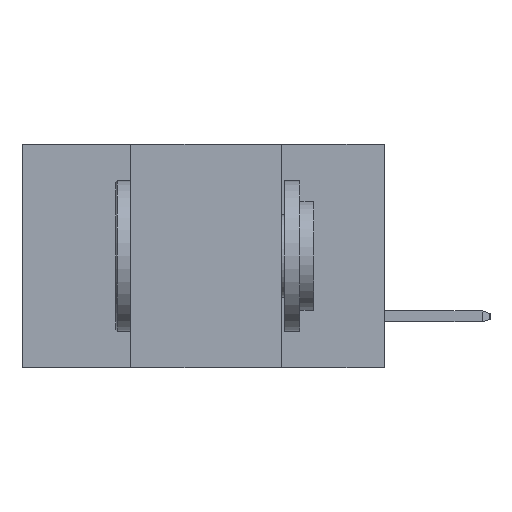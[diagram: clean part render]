
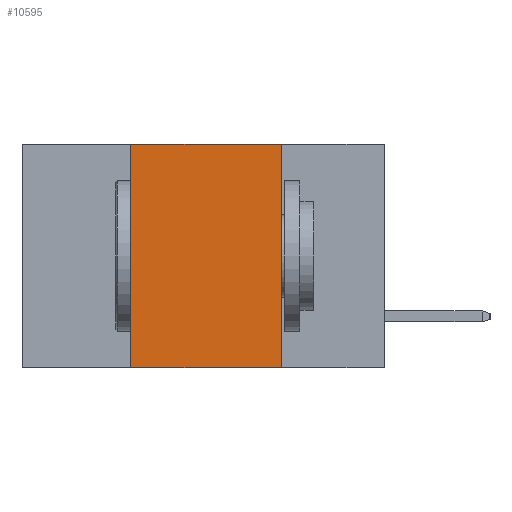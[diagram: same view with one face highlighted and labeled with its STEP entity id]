
A CAD part, left-side view. The second image highlights one B-rep face of the part: STEP entity #10595.
In plain terms, the highlighted planar face has unit normal (-1, 0, 0).
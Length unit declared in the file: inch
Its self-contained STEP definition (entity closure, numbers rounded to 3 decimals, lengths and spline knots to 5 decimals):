
#344 = ORIENTED_EDGE ( 'NONE', *, *, #7234, .F. ) ;
#406 = VERTEX_POINT ( 'NONE', #2446 ) ;
#418 = EDGE_CURVE ( 'NONE', #406, #7225, #11298, .T. ) ;
#929 = ORIENTED_EDGE ( 'NONE', *, *, #8746, .F. ) ;
#1268 = ORIENTED_EDGE ( 'NONE', *, *, #7599, .T. ) ;
#2446 = CARTESIAN_POINT ( 'NONE',  ( 0., 0.17, 0. ) ) ;
#2513 = LINE ( 'NONE', #8634, #9541 ) ;
#3117 = LINE ( 'NONE', #3710, #10073 ) ;
#3343 = DIRECTION ( 'NONE',  ( 0., -1., 0. ) ) ;
#3696 = CARTESIAN_POINT ( 'NONE',  ( 0., 0.17, 0. ) ) ;
#3710 = CARTESIAN_POINT ( 'NONE',  ( 0., 0.6, -0.37 ) ) ;
#3955 = AXIS2_PLACEMENT_3D ( 'NONE', #10281, #4976, #11161 ) ;
#4200 = VECTOR ( 'NONE', #10856, 39.37008 ) ;
#4884 = VECTOR ( 'NONE', #6830, 39.37008 ) ;
#4941 = PLANE ( 'NONE',  #3955 ) ;
#4976 = DIRECTION ( 'NONE',  ( 1., 0., 0. ) ) ;
#5404 = VERTEX_POINT ( 'NONE', #8110 ) ;
#6830 = DIRECTION ( 'NONE',  ( 0., 0., 1. ) ) ;
#7225 = VERTEX_POINT ( 'NONE', #9075 ) ;
#7234 = EDGE_CURVE ( 'NONE', #9835, #406, #2513, .T. ) ;
#7599 = EDGE_CURVE ( 'NONE', #5404, #7225, #3117, .T. ) ;
#8048 = ORIENTED_EDGE ( 'NONE', *, *, #418, .F. ) ;
#8110 = CARTESIAN_POINT ( 'NONE',  ( 0., 0.42, -0.37 ) ) ;
#8379 = CARTESIAN_POINT ( 'NONE',  ( 0., 0.42, 0. ) ) ;
#8573 = DIRECTION ( 'NONE',  ( 0., -1., 0. ) ) ;
#8634 = CARTESIAN_POINT ( 'NONE',  ( 0., 0.6, 0. ) ) ;
#8746 = EDGE_CURVE ( 'NONE', #5404, #9835, #9369, .T. ) ;
#9075 = CARTESIAN_POINT ( 'NONE',  ( 0., 0.17, -0.37 ) ) ;
#9369 = LINE ( 'NONE', #11200, #4884 ) ;
#9459 = FACE_OUTER_BOUND ( 'NONE', #11156, .T. ) ;
#9541 = VECTOR ( 'NONE', #8573, 39.37008 ) ;
#9835 = VERTEX_POINT ( 'NONE', #8379 ) ;
#10073 = VECTOR ( 'NONE', #3343, 39.37008 ) ;
#10281 = CARTESIAN_POINT ( 'NONE',  ( 0., 0.6, 0. ) ) ;
#10595 = ADVANCED_FACE ( 'NONE', ( #9459 ), #4941, .F. ) ;
#10856 = DIRECTION ( 'NONE',  ( 0., 0., -1. ) ) ;
#11156 = EDGE_LOOP ( 'NONE', ( #8048, #344, #929, #1268 ) ) ;
#11161 = DIRECTION ( 'NONE',  ( 0., 0., -1. ) ) ;
#11200 = CARTESIAN_POINT ( 'NONE',  ( 0., 0.42, 0. ) ) ;
#11298 = LINE ( 'NONE', #3696, #4200 ) ;
